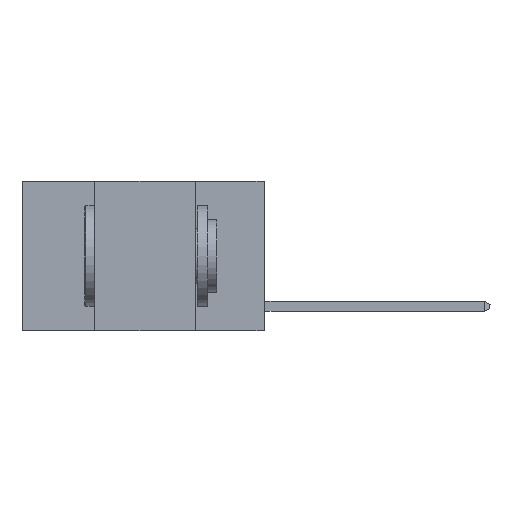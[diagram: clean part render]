
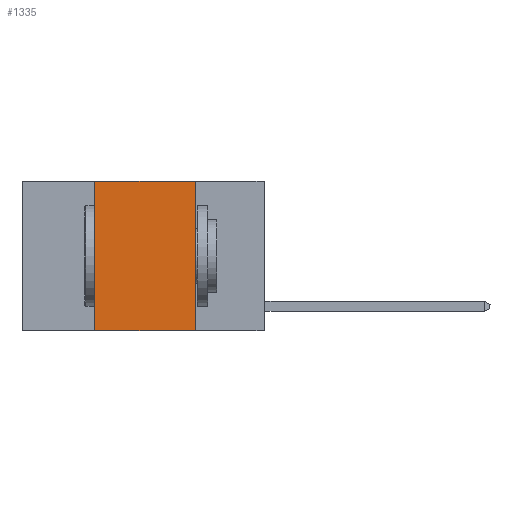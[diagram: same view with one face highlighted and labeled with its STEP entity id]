
A CAD part, left-side view. The second image highlights one B-rep face of the part: STEP entity #1335.
In plain terms, the highlighted planar face has unit normal (-1, 0, 0).
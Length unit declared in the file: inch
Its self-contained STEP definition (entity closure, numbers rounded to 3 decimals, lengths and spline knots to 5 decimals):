
#430 = DIRECTION ( 'NONE',  ( 0., 0., 1. ) ) ;
#655 = VECTOR ( 'NONE', #18204, 39.37008 ) ;
#1051 = CARTESIAN_POINT ( 'NONE',  ( 0., 0.6, 0. ) ) ;
#1335 = ADVANCED_FACE ( 'NONE', ( #21077 ), #23971, .F. ) ;
#1693 = DIRECTION ( 'NONE',  ( 1., 0., 0. ) ) ;
#1926 = VERTEX_POINT ( 'NONE', #26567 ) ;
#3913 = ORIENTED_EDGE ( 'NONE', *, *, #13590, .T. ) ;
#4688 = LINE ( 'NONE', #13524, #21747 ) ;
#6525 = LINE ( 'NONE', #1051, #13822 ) ;
#7573 = ORIENTED_EDGE ( 'NONE', *, *, #24535, .F. ) ;
#7930 = LINE ( 'NONE', #11614, #655 ) ;
#7969 = ORIENTED_EDGE ( 'NONE', *, *, #10427, .F. ) ;
#9574 = CARTESIAN_POINT ( 'NONE',  ( 0., 0.17, 0. ) ) ;
#9668 = ORIENTED_EDGE ( 'NONE', *, *, #23595, .F. ) ;
#10427 = EDGE_CURVE ( 'NONE', #21720, #11581, #20391, .T. ) ;
#11581 = VERTEX_POINT ( 'NONE', #11954 ) ;
#11614 = CARTESIAN_POINT ( 'NONE',  ( 0., 0.6, -0.37 ) ) ;
#11954 = CARTESIAN_POINT ( 'NONE',  ( 0., 0.17, -0.37 ) ) ;
#12354 = AXIS2_PLACEMENT_3D ( 'NONE', #28220, #1693, #14677 ) ;
#12488 = VERTEX_POINT ( 'NONE', #24541 ) ;
#13524 = CARTESIAN_POINT ( 'NONE',  ( 0., 0.42, 0. ) ) ;
#13590 = EDGE_CURVE ( 'NONE', #1926, #11581, #7930, .T. ) ;
#13822 = VECTOR ( 'NONE', #16783, 39.37008 ) ;
#14677 = DIRECTION ( 'NONE',  ( 0., 0., -1. ) ) ;
#15914 = DIRECTION ( 'NONE',  ( 0., 0., -1. ) ) ;
#16783 = DIRECTION ( 'NONE',  ( 0., -1., 0. ) ) ;
#17765 = CARTESIAN_POINT ( 'NONE',  ( 0., 0.17, 0. ) ) ;
#18204 = DIRECTION ( 'NONE',  ( 0., -1., 0. ) ) ;
#20391 = LINE ( 'NONE', #9574, #25629 ) ;
#21077 = FACE_OUTER_BOUND ( 'NONE', #22968, .T. ) ;
#21720 = VERTEX_POINT ( 'NONE', #17765 ) ;
#21747 = VECTOR ( 'NONE', #430, 39.37008 ) ;
#22968 = EDGE_LOOP ( 'NONE', ( #7969, #9668, #7573, #3913 ) ) ;
#23595 = EDGE_CURVE ( 'NONE', #12488, #21720, #6525, .T. ) ;
#23971 = PLANE ( 'NONE',  #12354 ) ;
#24535 = EDGE_CURVE ( 'NONE', #1926, #12488, #4688, .T. ) ;
#24541 = CARTESIAN_POINT ( 'NONE',  ( 0., 0.42, 0. ) ) ;
#25629 = VECTOR ( 'NONE', #15914, 39.37008 ) ;
#26567 = CARTESIAN_POINT ( 'NONE',  ( 0., 0.42, -0.37 ) ) ;
#28220 = CARTESIAN_POINT ( 'NONE',  ( 0., 0.6, 0. ) ) ;
